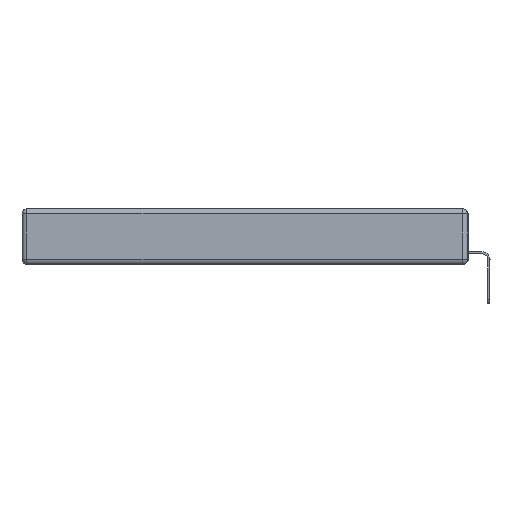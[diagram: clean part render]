
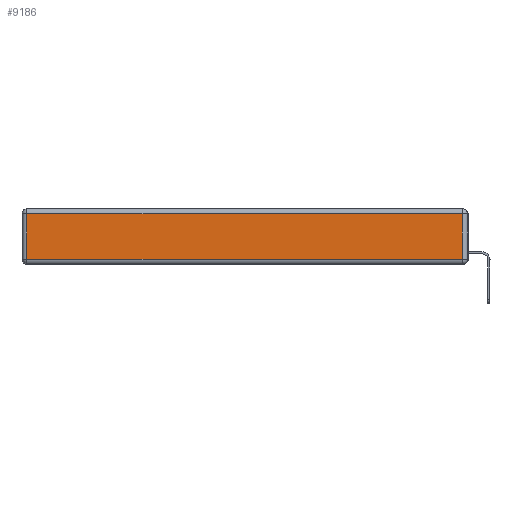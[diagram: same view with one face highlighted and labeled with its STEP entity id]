
A CAD part, left-side view. The second image highlights one B-rep face of the part: STEP entity #9186.
In plain terms, the highlighted planar face has unit normal (-1, 0, 0).
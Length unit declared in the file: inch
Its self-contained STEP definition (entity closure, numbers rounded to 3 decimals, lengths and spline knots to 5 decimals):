
#93 = PLANE ( 'NONE',  #7135 ) ;
#188 = CARTESIAN_POINT ( 'NONE',  ( 0., 0.03, -0.313 ) ) ;
#304 = ORIENTED_EDGE ( 'NONE', *, *, #1277, .T. ) ;
#995 = VERTEX_POINT ( 'NONE', #13287 ) ;
#1024 = DIRECTION ( 'NONE',  ( 0., 0., 1. ) ) ;
#1110 = CARTESIAN_POINT ( 'NONE',  ( 0., 0.03, -0.03 ) ) ;
#1277 = EDGE_CURVE ( 'NONE', #1429, #2192, #3688, .T. ) ;
#1429 = VERTEX_POINT ( 'NONE', #188 ) ;
#2192 = VERTEX_POINT ( 'NONE', #1110 ) ;
#3286 = LINE ( 'NONE', #9497, #7841 ) ;
#3688 = LINE ( 'NONE', #11523, #10221 ) ;
#3756 = EDGE_CURVE ( 'NONE', #995, #10620, #3286, .T. ) ;
#4054 = DIRECTION ( 'NONE',  ( 0., 0., 1. ) ) ;
#4235 = VECTOR ( 'NONE', #9033, 39.37008 ) ;
#4690 = ORIENTED_EDGE ( 'NONE', *, *, #3756, .T. ) ;
#6276 = ORIENTED_EDGE ( 'NONE', *, *, #13006, .T. ) ;
#6963 = LINE ( 'NONE', #8489, #10456 ) ;
#7135 = AXIS2_PLACEMENT_3D ( 'NONE', #10759, #12939, #1024 ) ;
#7841 = VECTOR ( 'NONE', #10724, 39.37008 ) ;
#7965 = CARTESIAN_POINT ( 'NONE',  ( 0., 0., -0.313 ) ) ;
#8489 = CARTESIAN_POINT ( 'NONE',  ( 0., 2.75, -0.03 ) ) ;
#9033 = DIRECTION ( 'NONE',  ( 0., -1., 0. ) ) ;
#9186 = ADVANCED_FACE ( 'NONE', ( #11059 ), #93, .T. ) ;
#9408 = EDGE_LOOP ( 'NONE', ( #6276, #304, #13758, #4690 ) ) ;
#9497 = CARTESIAN_POINT ( 'NONE',  ( 0., 2.72, -0.343 ) ) ;
#10151 = CARTESIAN_POINT ( 'NONE',  ( 0., 2.72, -0.313 ) ) ;
#10221 = VECTOR ( 'NONE', #4054, 39.37008 ) ;
#10456 = VECTOR ( 'NONE', #13750, 39.37008 ) ;
#10620 = VERTEX_POINT ( 'NONE', #10151 ) ;
#10724 = DIRECTION ( 'NONE',  ( 0., 0., -1. ) ) ;
#10759 = CARTESIAN_POINT ( 'NONE',  ( 0., 0., -0.343 ) ) ;
#11059 = FACE_OUTER_BOUND ( 'NONE', #9408, .T. ) ;
#11523 = CARTESIAN_POINT ( 'NONE',  ( 0., 0.03, -0.343 ) ) ;
#12673 = EDGE_CURVE ( 'NONE', #2192, #995, #6963, .T. ) ;
#12939 = DIRECTION ( 'NONE',  ( -1., 0., 0. ) ) ;
#13006 = EDGE_CURVE ( 'NONE', #10620, #1429, #13659, .T. ) ;
#13287 = CARTESIAN_POINT ( 'NONE',  ( 0., 2.72, -0.03 ) ) ;
#13659 = LINE ( 'NONE', #7965, #4235 ) ;
#13750 = DIRECTION ( 'NONE',  ( 0., 1., 0. ) ) ;
#13758 = ORIENTED_EDGE ( 'NONE', *, *, #12673, .T. ) ;
